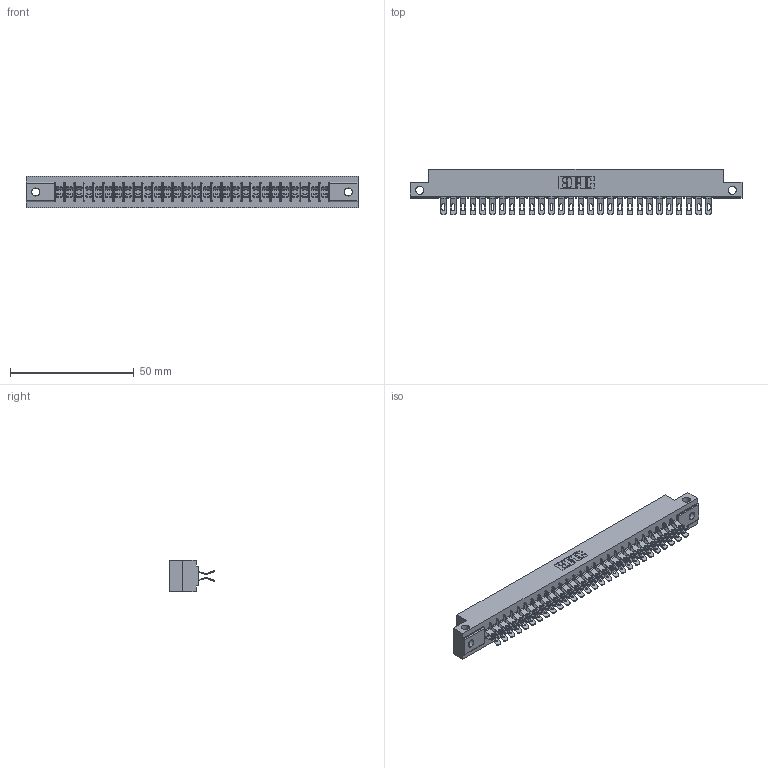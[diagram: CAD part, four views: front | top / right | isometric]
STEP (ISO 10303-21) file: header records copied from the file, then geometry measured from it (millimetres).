
FILE_DESCRIPTION (( 'STEP AP203' ), '1' );
FILE_NAME ('355-056-555-512.STEP', '2020-09-20T08:17:23', ( '' ), ( '' ), 'SwSTEP 2.0', 'SolidWorks 2020', '' );
FILE_SCHEMA (( 'CONFIG_CONTROL_DESIGN' ));
Length unit declared in the file: inch
Products named in the file (3): 305 Part_.128 Dia; 305-290-001_555; 355-056-555-512
Assembly tree (57 placements, depth 2):
  355-056-555-512
    305 Part_.128 Dia
    305-290-001_555  x56
Bounding box: 133.96 x 18.41 x 12.7 mm (x, y, z)
Volume: 13466.4 mm3; surface area: 18569.5 mm2
Topology: 57 solids, 57 shells, 3824 faces, 11412 edges, 7452 vertices
Faces by surface type: plane 1860, cylinder 1852, sphere 112
Entity records: 33051 total; most frequent: CARTESIAN_POINT 5536, ORIENTED_EDGE 5440, DIRECTION 5300, EDGE_CURVE 2720, VECTOR 2148, LINE 2148, VERTEX_POINT 1732, AXIS2_PLACEMENT_3D 1576
